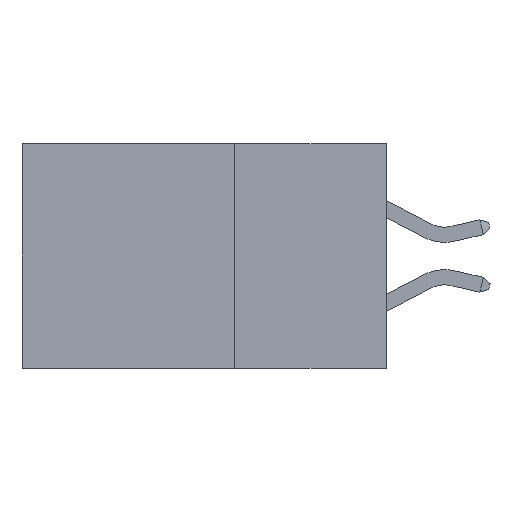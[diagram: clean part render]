
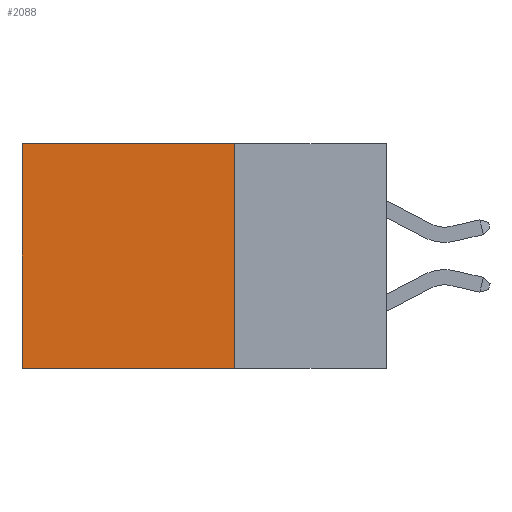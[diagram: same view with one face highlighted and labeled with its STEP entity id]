
A CAD part, left-side view. The second image highlights one B-rep face of the part: STEP entity #2088.
In plain terms, the highlighted planar face has unit normal (-1, 0, 0).
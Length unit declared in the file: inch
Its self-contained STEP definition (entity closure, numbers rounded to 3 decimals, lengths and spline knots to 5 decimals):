
#750 = VECTOR ( 'NONE', #12125, 39.37008 ) ;
#1424 = CARTESIAN_POINT ( 'NONE',  ( 0.298, 0.6, 0. ) ) ;
#1517 = DIRECTION ( 'NONE',  ( 0., 1., 0. ) ) ;
#2088 = ADVANCED_FACE ( 'NONE', ( #29337 ), #6162, .F. ) ;
#4094 = EDGE_CURVE ( 'NONE', #15830, #24486, #6954, .T. ) ;
#6162 = PLANE ( 'NONE',  #19850 ) ;
#6954 = LINE ( 'NONE', #23739, #750 ) ;
#7763 = EDGE_LOOP ( 'NONE', ( #19246, #10904, #19939, #18549 ) ) ;
#8702 = CARTESIAN_POINT ( 'NONE',  ( 0.298, 0.25, -0.37 ) ) ;
#9160 = LINE ( 'NONE', #24269, #17544 ) ;
#10035 = LINE ( 'NONE', #22055, #14763 ) ;
#10904 = ORIENTED_EDGE ( 'NONE', *, *, #24201, .F. ) ;
#12125 = DIRECTION ( 'NONE',  ( 0., 0., -1. ) ) ;
#13359 = CARTESIAN_POINT ( 'NONE',  ( 0.298, 0.25, 0. ) ) ;
#14693 = VERTEX_POINT ( 'NONE', #8702 ) ;
#14763 = VECTOR ( 'NONE', #17248, 39.37008 ) ;
#15082 = EDGE_CURVE ( 'NONE', #15273, #14693, #10035, .T. ) ;
#15123 = CARTESIAN_POINT ( 'NONE',  ( 0.298, 0.25, -0.37 ) ) ;
#15273 = VERTEX_POINT ( 'NONE', #22454 ) ;
#15680 = VECTOR ( 'NONE', #1517, 39.37008 ) ;
#15830 = VERTEX_POINT ( 'NONE', #1424 ) ;
#17248 = DIRECTION ( 'NONE',  ( 0., 0., -1. ) ) ;
#17544 = VECTOR ( 'NONE', #26317, 39.37008 ) ;
#17809 = EDGE_CURVE ( 'NONE', #15273, #15830, #9160, .T. ) ;
#18549 = ORIENTED_EDGE ( 'NONE', *, *, #17809, .T. ) ;
#18784 = CARTESIAN_POINT ( 'NONE',  ( 0.298, 0.6, -0.37 ) ) ;
#19246 = ORIENTED_EDGE ( 'NONE', *, *, #4094, .T. ) ;
#19850 = AXIS2_PLACEMENT_3D ( 'NONE', #13359, #22833, #27435 ) ;
#19939 = ORIENTED_EDGE ( 'NONE', *, *, #15082, .F. ) ;
#22055 = CARTESIAN_POINT ( 'NONE',  ( 0.298, 0.25, 0. ) ) ;
#22454 = CARTESIAN_POINT ( 'NONE',  ( 0.298, 0.25, 0. ) ) ;
#22833 = DIRECTION ( 'NONE',  ( 1., 0., 0. ) ) ;
#23739 = CARTESIAN_POINT ( 'NONE',  ( 0.298, 0.6, 0. ) ) ;
#24201 = EDGE_CURVE ( 'NONE', #14693, #24486, #25157, .T. ) ;
#24269 = CARTESIAN_POINT ( 'NONE',  ( 0.298, 0.25, 0. ) ) ;
#24486 = VERTEX_POINT ( 'NONE', #18784 ) ;
#25157 = LINE ( 'NONE', #15123, #15680 ) ;
#26317 = DIRECTION ( 'NONE',  ( 0., 1., 0. ) ) ;
#27435 = DIRECTION ( 'NONE',  ( 0., 0., -1. ) ) ;
#29337 = FACE_OUTER_BOUND ( 'NONE', #7763, .T. ) ;
